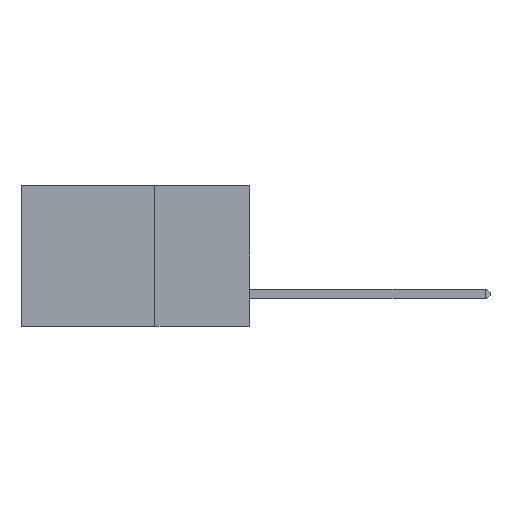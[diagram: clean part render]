
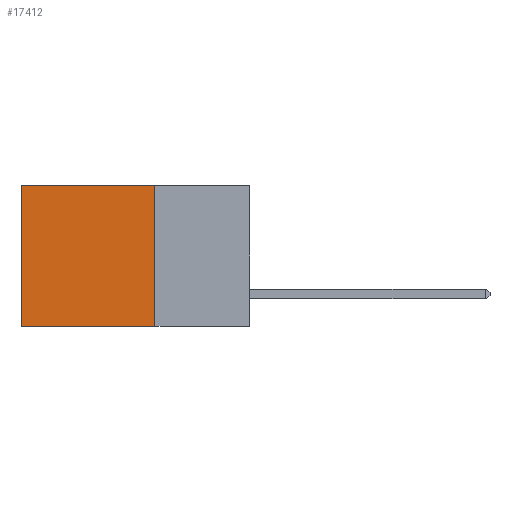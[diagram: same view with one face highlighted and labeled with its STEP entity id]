
A CAD part, left-side view. The second image highlights one B-rep face of the part: STEP entity #17412.
In plain terms, the highlighted planar face has unit normal (-1, 0, 0).
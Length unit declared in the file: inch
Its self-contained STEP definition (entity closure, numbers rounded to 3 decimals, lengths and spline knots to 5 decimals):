
#541 = VERTEX_POINT ( 'NONE', #12620 ) ;
#990 = ORIENTED_EDGE ( 'NONE', *, *, #6890, .T. ) ;
#1371 = LINE ( 'NONE', #19469, #14055 ) ;
#1753 = DIRECTION ( 'NONE',  ( 0., 1., 0. ) ) ;
#2314 = ORIENTED_EDGE ( 'NONE', *, *, #17549, .F. ) ;
#3518 = CARTESIAN_POINT ( 'NONE',  ( 0.2875, 0.25, 0. ) ) ;
#3550 = ORIENTED_EDGE ( 'NONE', *, *, #12711, .F. ) ;
#3922 = CARTESIAN_POINT ( 'NONE',  ( 0.2875, 0.6, 0. ) ) ;
#4001 = DIRECTION ( 'NONE',  ( 0., 0., -1. ) ) ;
#4775 = VERTEX_POINT ( 'NONE', #8874 ) ;
#5195 = DIRECTION ( 'NONE',  ( 0., 1., 0. ) ) ;
#5333 = DIRECTION ( 'NONE',  ( 0., 0., -1. ) ) ;
#5902 = LINE ( 'NONE', #3518, #14058 ) ;
#6294 = EDGE_LOOP ( 'NONE', ( #990, #3550, #2314, #10490 ) ) ;
#6715 = CARTESIAN_POINT ( 'NONE',  ( 0.2875, 0.25, 0. ) ) ;
#6801 = VECTOR ( 'NONE', #5333, 39.37008 ) ;
#6890 = EDGE_CURVE ( 'NONE', #4775, #541, #16140, .T. ) ;
#8020 = CARTESIAN_POINT ( 'NONE',  ( 0.2875, 0.25, -0.37 ) ) ;
#8386 = DIRECTION ( 'NONE',  ( 0., 0., -1. ) ) ;
#8457 = VERTEX_POINT ( 'NONE', #8020 ) ;
#8874 = CARTESIAN_POINT ( 'NONE',  ( 0.2875, 0.6, 0. ) ) ;
#9304 = CARTESIAN_POINT ( 'NONE',  ( 0.2875, 0.25, 0. ) ) ;
#9967 = PLANE ( 'NONE',  #13019 ) ;
#10490 = ORIENTED_EDGE ( 'NONE', *, *, #14025, .T. ) ;
#12620 = CARTESIAN_POINT ( 'NONE',  ( 0.2875, 0.6, -0.37 ) ) ;
#12711 = EDGE_CURVE ( 'NONE', #8457, #541, #1371, .T. ) ;
#13019 = AXIS2_PLACEMENT_3D ( 'NONE', #6715, #17930, #8386 ) ;
#13218 = FACE_OUTER_BOUND ( 'NONE', #6294, .T. ) ;
#13626 = CARTESIAN_POINT ( 'NONE',  ( 0.2875, 0.25, 0. ) ) ;
#14025 = EDGE_CURVE ( 'NONE', #18525, #4775, #5902, .T. ) ;
#14055 = VECTOR ( 'NONE', #1753, 39.37008 ) ;
#14058 = VECTOR ( 'NONE', #5195, 39.37008 ) ;
#15387 = LINE ( 'NONE', #13626, #6801 ) ;
#16140 = LINE ( 'NONE', #3922, #20278 ) ;
#17412 = ADVANCED_FACE ( 'NONE', ( #13218 ), #9967, .F. ) ;
#17549 = EDGE_CURVE ( 'NONE', #18525, #8457, #15387, .T. ) ;
#17930 = DIRECTION ( 'NONE',  ( 1., 0., 0. ) ) ;
#18525 = VERTEX_POINT ( 'NONE', #9304 ) ;
#19469 = CARTESIAN_POINT ( 'NONE',  ( 0.2875, 0.25, -0.37 ) ) ;
#20278 = VECTOR ( 'NONE', #4001, 39.37008 ) ;
